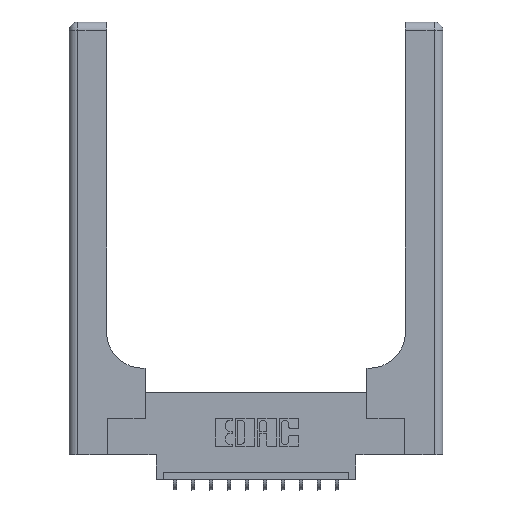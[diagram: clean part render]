
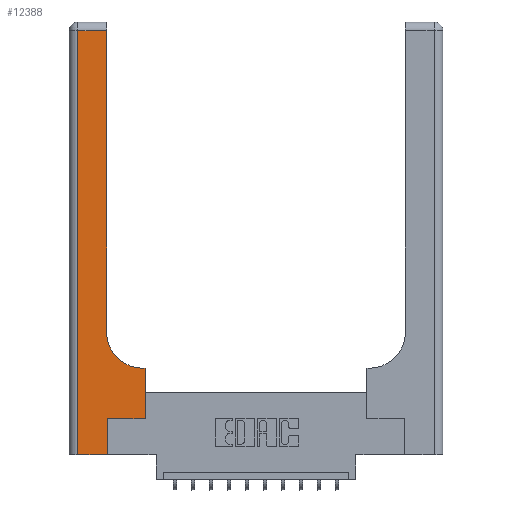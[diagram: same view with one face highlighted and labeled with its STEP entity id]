
A CAD part, top view. The second image highlights one B-rep face of the part: STEP entity #12388.
In plain terms, the highlighted planar face has unit normal (0, 0, 1).
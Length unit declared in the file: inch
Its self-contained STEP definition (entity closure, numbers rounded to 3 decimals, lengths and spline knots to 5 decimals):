
#21 = CARTESIAN_POINT ( 'NONE',  ( 0.528, 0.25, 0.37 ) ) ;
#251 = EDGE_CURVE ( 'NONE', #2806, #1265, #3510, .T. ) ;
#312 = DIRECTION ( 'NONE',  ( 1., 0., 0. ) ) ;
#348 = LINE ( 'NONE', #5297, #10213 ) ;
#368 = VECTOR ( 'NONE', #11739, 39.37008 ) ;
#379 = ORIENTED_EDGE ( 'NONE', *, *, #1138, .T. ) ;
#437 = EDGE_CURVE ( 'NONE', #15084, #2806, #2855, .T. ) ;
#672 = LINE ( 'NONE', #7029, #14295 ) ;
#975 = DIRECTION ( 'NONE',  ( -1., 0., 0. ) ) ;
#998 = DIRECTION ( 'NONE',  ( -1., 0., 0. ) ) ;
#1138 = EDGE_CURVE ( 'NONE', #10283, #10296, #2402, .T. ) ;
#1265 = VERTEX_POINT ( 'NONE', #7841 ) ;
#1346 = DIRECTION ( 'NONE',  ( 0., 1., 0. ) ) ;
#2270 = VERTEX_POINT ( 'NONE', #16311 ) ;
#2402 = LINE ( 'NONE', #13579, #12619 ) ;
#2645 = AXIS2_PLACEMENT_3D ( 'NONE', #12298, #12211, #6144 ) ;
#2806 = VERTEX_POINT ( 'NONE', #7904 ) ;
#2855 = LINE ( 'NONE', #10226, #8521 ) ;
#2914 = EDGE_CURVE ( 'NONE', #1265, #7464, #672, .T. ) ;
#3381 = VECTOR ( 'NONE', #8491, 39.37008 ) ;
#3510 = LINE ( 'NONE', #8711, #9038 ) ;
#3829 = CARTESIAN_POINT ( 'NONE',  ( 0.06, 0., 0.37 ) ) ;
#4151 = VERTEX_POINT ( 'NONE', #13349 ) ;
#4195 = EDGE_CURVE ( 'NONE', #15836, #4151, #13214, .T. ) ;
#5158 = LINE ( 'NONE', #12870, #14583 ) ;
#5297 = CARTESIAN_POINT ( 'NONE',  ( 0.26, 3., 0.37 ) ) ;
#5748 = CARTESIAN_POINT ( 'NONE',  ( 0.51, 0.6, 0.37 ) ) ;
#5949 = CARTESIAN_POINT ( 'NONE',  ( 0.528, 0.25, 0.37 ) ) ;
#6093 = FACE_OUTER_BOUND ( 'NONE', #14814, .T. ) ;
#6132 = ORIENTED_EDGE ( 'NONE', *, *, #4195, .T. ) ;
#6144 = DIRECTION ( 'NONE',  ( 1., 0., 0. ) ) ;
#6174 = ORIENTED_EDGE ( 'NONE', *, *, #251, .T. ) ;
#6581 = AXIS2_PLACEMENT_3D ( 'NONE', #8393, #7262, #975 ) ;
#7029 = CARTESIAN_POINT ( 'NONE',  ( 0.265, 0.25, 0.37 ) ) ;
#7131 = CARTESIAN_POINT ( 'NONE',  ( 0.26, 2.94, 0.37 ) ) ;
#7262 = DIRECTION ( 'NONE',  ( 0., 0., -1. ) ) ;
#7354 = ORIENTED_EDGE ( 'NONE', *, *, #437, .T. ) ;
#7464 = VERTEX_POINT ( 'NONE', #21 ) ;
#7710 = EDGE_CURVE ( 'NONE', #7464, #2270, #14893, .T. ) ;
#7811 = ORIENTED_EDGE ( 'NONE', *, *, #9436, .T. ) ;
#7841 = CARTESIAN_POINT ( 'NONE',  ( 0.265, 0.25, 0.37 ) ) ;
#7904 = CARTESIAN_POINT ( 'NONE',  ( 0.265, 0., 0.37 ) ) ;
#8212 = LINE ( 'NONE', #9457, #368 ) ;
#8393 = CARTESIAN_POINT ( 'NONE',  ( 0., 3., 0.37 ) ) ;
#8491 = DIRECTION ( 'NONE',  ( 0., 1., 0. ) ) ;
#8521 = VECTOR ( 'NONE', #312, 39.37008 ) ;
#8552 = EDGE_CURVE ( 'NONE', #4151, #10283, #348, .T. ) ;
#8557 = PLANE ( 'NONE',  #6581 ) ;
#8589 = CARTESIAN_POINT ( 'NONE',  ( 0.06, 2.94, 0.37 ) ) ;
#8711 = CARTESIAN_POINT ( 'NONE',  ( 0.265, 0., 0.37 ) ) ;
#9038 = VECTOR ( 'NONE', #16180, 39.37008 ) ;
#9076 = ORIENTED_EDGE ( 'NONE', *, *, #2914, .T. ) ;
#9436 = EDGE_CURVE ( 'NONE', #10296, #15084, #8212, .T. ) ;
#9457 = CARTESIAN_POINT ( 'NONE',  ( 0.06, 3., 0.37 ) ) ;
#10213 = VECTOR ( 'NONE', #1346, 39.37008 ) ;
#10226 = CARTESIAN_POINT ( 'NONE',  ( 0., 0., 0.37 ) ) ;
#10283 = VERTEX_POINT ( 'NONE', #7131 ) ;
#10296 = VERTEX_POINT ( 'NONE', #8589 ) ;
#10582 = ORIENTED_EDGE ( 'NONE', *, *, #8552, .T. ) ;
#11077 = ORIENTED_EDGE ( 'NONE', *, *, #7710, .T. ) ;
#11484 = DIRECTION ( 'NONE',  ( -1., 0., 0. ) ) ;
#11739 = DIRECTION ( 'NONE',  ( 0., -1., 0. ) ) ;
#12211 = DIRECTION ( 'NONE',  ( 0., 0., -1. ) ) ;
#12298 = CARTESIAN_POINT ( 'NONE',  ( 0.51, 0.85, 0.37 ) ) ;
#12388 = ADVANCED_FACE ( 'NONE', ( #6093 ), #8557, .F. ) ;
#12619 = VECTOR ( 'NONE', #998, 39.37008 ) ;
#12870 = CARTESIAN_POINT ( 'NONE',  ( 0.26, 0.6, 0.37 ) ) ;
#13214 = CIRCLE ( 'NONE', #2645, 0.25 ) ;
#13349 = CARTESIAN_POINT ( 'NONE',  ( 0.26, 0.85, 0.37 ) ) ;
#13579 = CARTESIAN_POINT ( 'NONE',  ( 0., 2.94, 0.37 ) ) ;
#14234 = ORIENTED_EDGE ( 'NONE', *, *, #14941, .T. ) ;
#14295 = VECTOR ( 'NONE', #14501, 39.37008 ) ;
#14501 = DIRECTION ( 'NONE',  ( 1., 0., 0. ) ) ;
#14583 = VECTOR ( 'NONE', #11484, 39.37008 ) ;
#14814 = EDGE_LOOP ( 'NONE', ( #10582, #379, #7811, #7354, #6174, #9076, #11077, #14234, #6132 ) ) ;
#14893 = LINE ( 'NONE', #5949, #3381 ) ;
#14941 = EDGE_CURVE ( 'NONE', #2270, #15836, #5158, .T. ) ;
#15084 = VERTEX_POINT ( 'NONE', #3829 ) ;
#15836 = VERTEX_POINT ( 'NONE', #5748 ) ;
#16180 = DIRECTION ( 'NONE',  ( 0., 1., 0. ) ) ;
#16311 = CARTESIAN_POINT ( 'NONE',  ( 0.528, 0.6, 0.37 ) ) ;
